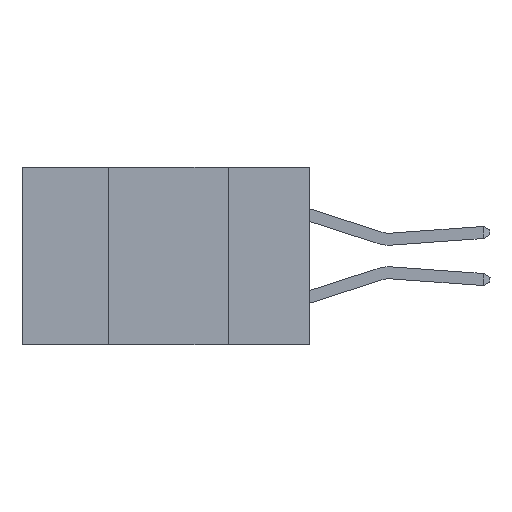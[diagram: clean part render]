
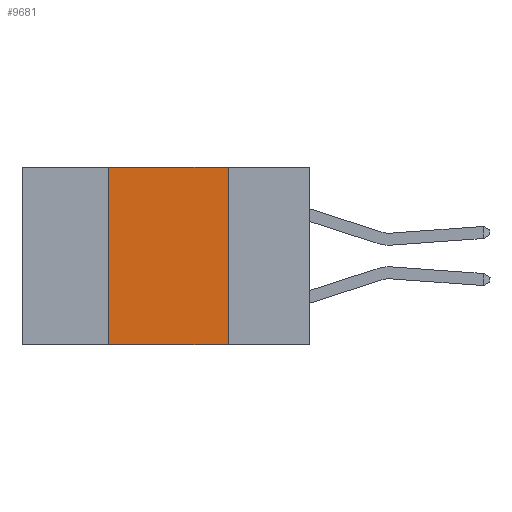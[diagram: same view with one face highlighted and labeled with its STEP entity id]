
A CAD part, left-side view. The second image highlights one B-rep face of the part: STEP entity #9681.
In plain terms, the highlighted planar face has unit normal (-1, 0, 0).
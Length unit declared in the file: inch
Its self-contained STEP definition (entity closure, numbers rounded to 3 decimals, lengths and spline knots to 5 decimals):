
#896 = DIRECTION ( 'NONE',  ( 0., 0., -1. ) ) ;
#1100 = LINE ( 'NONE', #1229, #11270 ) ;
#1229 = CARTESIAN_POINT ( 'NONE',  ( 0., 0.42, -0.37 ) ) ;
#1267 = DIRECTION ( 'NONE',  ( 0., -1., 0. ) ) ;
#1910 = ORIENTED_EDGE ( 'NONE', *, *, #2966, .F. ) ;
#2168 = VERTEX_POINT ( 'NONE', #11193 ) ;
#2321 = AXIS2_PLACEMENT_3D ( 'NONE', #5563, #3192, #7609 ) ;
#2788 = CARTESIAN_POINT ( 'NONE',  ( 0., 0.6, 0. ) ) ;
#2966 = EDGE_CURVE ( 'NONE', #11469, #8661, #1100, .T. ) ;
#3192 = DIRECTION ( 'NONE',  ( 1., 0., 0. ) ) ;
#4017 = CARTESIAN_POINT ( 'NONE',  ( 0., 0.17, -0.37 ) ) ;
#4377 = ORIENTED_EDGE ( 'NONE', *, *, #10769, .F. ) ;
#4403 = VECTOR ( 'NONE', #896, 39.37008 ) ;
#4483 = ORIENTED_EDGE ( 'NONE', *, *, #7815, .T. ) ;
#4763 = LINE ( 'NONE', #2788, #9210 ) ;
#4903 = CARTESIAN_POINT ( 'NONE',  ( 0., 0.42, 0. ) ) ;
#4930 = LINE ( 'NONE', #7456, #8799 ) ;
#5563 = CARTESIAN_POINT ( 'NONE',  ( 0., 0.6, 0. ) ) ;
#6072 = EDGE_CURVE ( 'NONE', #2168, #9350, #8572, .T. ) ;
#6620 = DIRECTION ( 'NONE',  ( 0., 0., 1. ) ) ;
#7456 = CARTESIAN_POINT ( 'NONE',  ( 0., 0.6, -0.37 ) ) ;
#7541 = ORIENTED_EDGE ( 'NONE', *, *, #6072, .F. ) ;
#7609 = DIRECTION ( 'NONE',  ( 0., 0., -1. ) ) ;
#7815 = EDGE_CURVE ( 'NONE', #11469, #9350, #4930, .T. ) ;
#8193 = PLANE ( 'NONE',  #2321 ) ;
#8572 = LINE ( 'NONE', #11404, #4403 ) ;
#8661 = VERTEX_POINT ( 'NONE', #4903 ) ;
#8799 = VECTOR ( 'NONE', #1267, 39.37008 ) ;
#9210 = VECTOR ( 'NONE', #10888, 39.37008 ) ;
#9350 = VERTEX_POINT ( 'NONE', #4017 ) ;
#9681 = ADVANCED_FACE ( 'NONE', ( #10048 ), #8193, .F. ) ;
#9810 = EDGE_LOOP ( 'NONE', ( #7541, #4377, #1910, #4483 ) ) ;
#10048 = FACE_OUTER_BOUND ( 'NONE', #9810, .T. ) ;
#10769 = EDGE_CURVE ( 'NONE', #8661, #2168, #4763, .T. ) ;
#10888 = DIRECTION ( 'NONE',  ( 0., -1., 0. ) ) ;
#11193 = CARTESIAN_POINT ( 'NONE',  ( 0., 0.17, 0. ) ) ;
#11250 = CARTESIAN_POINT ( 'NONE',  ( 0., 0.42, -0.37 ) ) ;
#11270 = VECTOR ( 'NONE', #6620, 39.37008 ) ;
#11404 = CARTESIAN_POINT ( 'NONE',  ( 0., 0.17, -0.37 ) ) ;
#11469 = VERTEX_POINT ( 'NONE', #11250 ) ;
